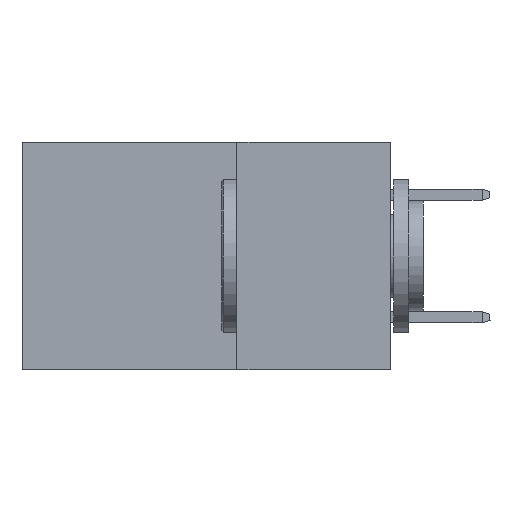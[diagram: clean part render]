
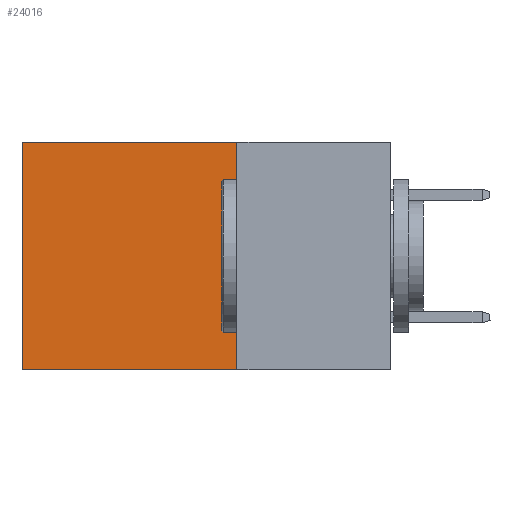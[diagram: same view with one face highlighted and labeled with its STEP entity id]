
A CAD part, left-side view. The second image highlights one B-rep face of the part: STEP entity #24016.
In plain terms, the highlighted planar face has unit normal (-1, 0, 0).
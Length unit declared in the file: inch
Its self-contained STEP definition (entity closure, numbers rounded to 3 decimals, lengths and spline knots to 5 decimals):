
#299 = CARTESIAN_POINT ( 'NONE',  ( 0.2875, 0.25, -0.37 ) ) ;
#323 = VERTEX_POINT ( 'NONE', #24057 ) ;
#2487 = CARTESIAN_POINT ( 'NONE',  ( 0.2875, 0.6, 0. ) ) ;
#4231 = DIRECTION ( 'NONE',  ( 0., 0., -1. ) ) ;
#5994 = CARTESIAN_POINT ( 'NONE',  ( 0.2875, 0.25, -0.37 ) ) ;
#6533 = DIRECTION ( 'NONE',  ( 0., 1., 0. ) ) ;
#6797 = ORIENTED_EDGE ( 'NONE', *, *, #28562, .F. ) ;
#6924 = LINE ( 'NONE', #5994, #17306 ) ;
#7957 = AXIS2_PLACEMENT_3D ( 'NONE', #26545, #28263, #17234 ) ;
#8071 = ORIENTED_EDGE ( 'NONE', *, *, #26932, .F. ) ;
#8210 = CARTESIAN_POINT ( 'NONE',  ( 0.2875, 0.25, 0. ) ) ;
#8561 = ORIENTED_EDGE ( 'NONE', *, *, #17075, .T. ) ;
#10139 = DIRECTION ( 'NONE',  ( 0., 1., 0. ) ) ;
#11022 = PLANE ( 'NONE',  #7957 ) ;
#11147 = FACE_OUTER_BOUND ( 'NONE', #14227, .T. ) ;
#11950 = VECTOR ( 'NONE', #6533, 39.37008 ) ;
#12474 = DIRECTION ( 'NONE',  ( 0., 0., -1. ) ) ;
#13138 = EDGE_CURVE ( 'NONE', #25925, #323, #22312, .T. ) ;
#13782 = VERTEX_POINT ( 'NONE', #299 ) ;
#14227 = EDGE_LOOP ( 'NONE', ( #8561, #6797, #8071, #15129 ) ) ;
#14470 = VECTOR ( 'NONE', #4231, 39.37008 ) ;
#15129 = ORIENTED_EDGE ( 'NONE', *, *, #13138, .T. ) ;
#16516 = LINE ( 'NONE', #2487, #14470 ) ;
#17075 = EDGE_CURVE ( 'NONE', #323, #26613, #16516, .T. ) ;
#17234 = DIRECTION ( 'NONE',  ( 0., 0., -1. ) ) ;
#17306 = VECTOR ( 'NONE', #10139, 39.37008 ) ;
#19949 = CARTESIAN_POINT ( 'NONE',  ( 0.2875, 0.25, 0. ) ) ;
#21236 = VECTOR ( 'NONE', #12474, 39.37008 ) ;
#22312 = LINE ( 'NONE', #23977, #11950 ) ;
#22622 = LINE ( 'NONE', #8210, #21236 ) ;
#23977 = CARTESIAN_POINT ( 'NONE',  ( 0.2875, 0.25, 0. ) ) ;
#24016 = ADVANCED_FACE ( 'NONE', ( #11147 ), #11022, .F. ) ;
#24057 = CARTESIAN_POINT ( 'NONE',  ( 0.2875, 0.6, 0. ) ) ;
#24876 = CARTESIAN_POINT ( 'NONE',  ( 0.2875, 0.6, -0.37 ) ) ;
#25925 = VERTEX_POINT ( 'NONE', #19949 ) ;
#26545 = CARTESIAN_POINT ( 'NONE',  ( 0.2875, 0.25, 0. ) ) ;
#26613 = VERTEX_POINT ( 'NONE', #24876 ) ;
#26932 = EDGE_CURVE ( 'NONE', #25925, #13782, #22622, .T. ) ;
#28263 = DIRECTION ( 'NONE',  ( 1., 0., 0. ) ) ;
#28562 = EDGE_CURVE ( 'NONE', #13782, #26613, #6924, .T. ) ;
